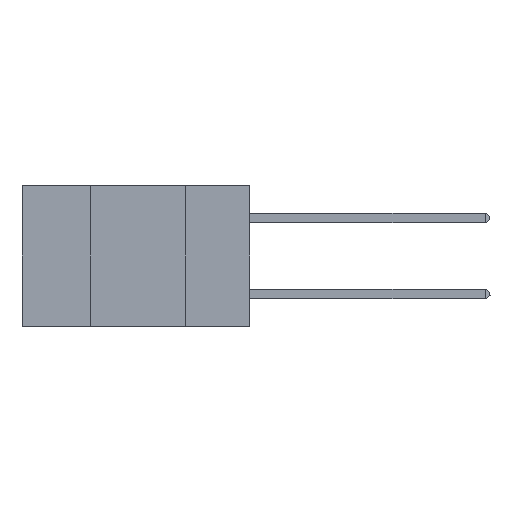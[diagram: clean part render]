
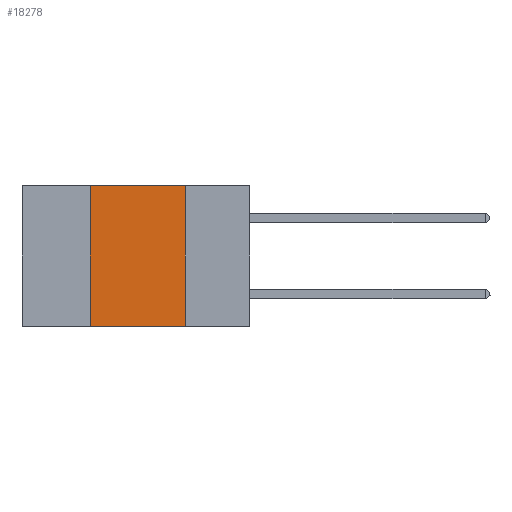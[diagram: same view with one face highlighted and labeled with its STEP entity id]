
A CAD part, left-side view. The second image highlights one B-rep face of the part: STEP entity #18278.
In plain terms, the highlighted planar face has unit normal (-1, 0, 0).
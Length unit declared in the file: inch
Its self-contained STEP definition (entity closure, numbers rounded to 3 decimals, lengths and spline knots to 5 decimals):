
#232 = EDGE_CURVE ( 'NONE', #23510, #14868, #25287, .T. ) ;
#295 = EDGE_CURVE ( 'NONE', #14868, #11281, #12838, .T. ) ;
#724 = FACE_OUTER_BOUND ( 'NONE', #25571, .T. ) ;
#2992 = VECTOR ( 'NONE', #4681, 39.37008 ) ;
#3895 = PLANE ( 'NONE',  #18178 ) ;
#4585 = CARTESIAN_POINT ( 'NONE',  ( 0., 0.6, 0. ) ) ;
#4681 = DIRECTION ( 'NONE',  ( 0., 0., -1. ) ) ;
#6736 = CARTESIAN_POINT ( 'NONE',  ( 0., 0.6, -0.37 ) ) ;
#7237 = CARTESIAN_POINT ( 'NONE',  ( 0., 0.42, 0. ) ) ;
#7664 = VECTOR ( 'NONE', #21379, 39.37008 ) ;
#8271 = EDGE_CURVE ( 'NONE', #15724, #23510, #8894, .T. ) ;
#8549 = ORIENTED_EDGE ( 'NONE', *, *, #295, .F. ) ;
#8894 = LINE ( 'NONE', #7237, #9209 ) ;
#9209 = VECTOR ( 'NONE', #11444, 39.37008 ) ;
#11281 = VERTEX_POINT ( 'NONE', #23672 ) ;
#11356 = CARTESIAN_POINT ( 'NONE',  ( 0., 0.42, 0. ) ) ;
#11444 = DIRECTION ( 'NONE',  ( 0., 0., 1. ) ) ;
#11888 = ORIENTED_EDGE ( 'NONE', *, *, #8271, .F. ) ;
#12838 = LINE ( 'NONE', #21450, #2992 ) ;
#13334 = EDGE_CURVE ( 'NONE', #15724, #11281, #20072, .T. ) ;
#14079 = DIRECTION ( 'NONE',  ( 1., 0., 0. ) ) ;
#14868 = VERTEX_POINT ( 'NONE', #15017 ) ;
#15017 = CARTESIAN_POINT ( 'NONE',  ( 0., 0.17, 0. ) ) ;
#15724 = VERTEX_POINT ( 'NONE', #22242 ) ;
#15945 = ORIENTED_EDGE ( 'NONE', *, *, #13334, .T. ) ;
#18178 = AXIS2_PLACEMENT_3D ( 'NONE', #22582, #14079, #24876 ) ;
#18278 = ADVANCED_FACE ( 'NONE', ( #724 ), #3895, .F. ) ;
#19256 = DIRECTION ( 'NONE',  ( 0., -1., 0. ) ) ;
#19715 = VECTOR ( 'NONE', #19256, 39.37008 ) ;
#20072 = LINE ( 'NONE', #6736, #7664 ) ;
#21379 = DIRECTION ( 'NONE',  ( 0., -1., 0. ) ) ;
#21450 = CARTESIAN_POINT ( 'NONE',  ( 0., 0.17, 0. ) ) ;
#22242 = CARTESIAN_POINT ( 'NONE',  ( 0., 0.42, -0.37 ) ) ;
#22582 = CARTESIAN_POINT ( 'NONE',  ( 0., 0.6, 0. ) ) ;
#23510 = VERTEX_POINT ( 'NONE', #11356 ) ;
#23672 = CARTESIAN_POINT ( 'NONE',  ( 0., 0.17, -0.37 ) ) ;
#24679 = ORIENTED_EDGE ( 'NONE', *, *, #232, .F. ) ;
#24876 = DIRECTION ( 'NONE',  ( 0., 0., -1. ) ) ;
#25287 = LINE ( 'NONE', #4585, #19715 ) ;
#25571 = EDGE_LOOP ( 'NONE', ( #8549, #24679, #11888, #15945 ) ) ;
